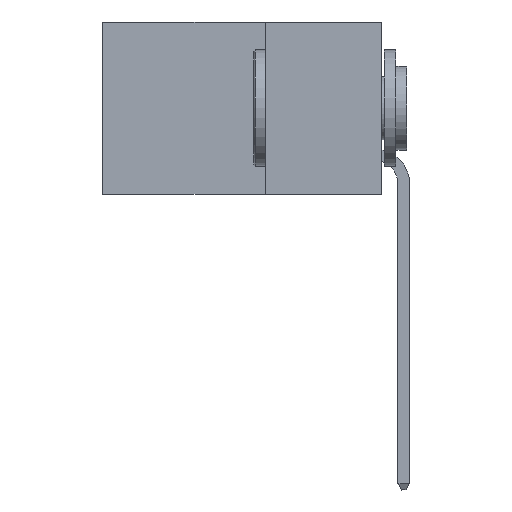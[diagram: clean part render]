
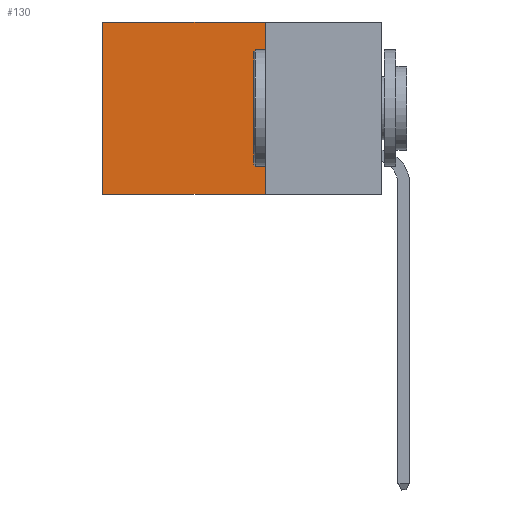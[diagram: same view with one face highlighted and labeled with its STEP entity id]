
A CAD part, left-side view. The second image highlights one B-rep face of the part: STEP entity #130.
In plain terms, the highlighted planar face has unit normal (-1, 0, 0).
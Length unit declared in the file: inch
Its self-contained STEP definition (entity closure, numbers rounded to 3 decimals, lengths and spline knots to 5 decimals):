
#66 = FACE_OUTER_BOUND ( 'NONE', #1054, .T. ) ;
#108 = CARTESIAN_POINT ( 'NONE',  ( 0.2875, 0.6, -0.37 ) ) ;
#113 = DIRECTION ( 'NONE',  ( 0., 1., 0. ) ) ;
#130 = ADVANCED_FACE ( 'NONE', ( #66 ), #8035, .F. ) ;
#578 = LINE ( 'NONE', #3167, #718 ) ;
#718 = VECTOR ( 'NONE', #9207, 39.37008 ) ;
#1054 = EDGE_LOOP ( 'NONE', ( #7247, #6273, #2161, #7801 ) ) ;
#1156 = CARTESIAN_POINT ( 'NONE',  ( 0.2875, 0.25, 0. ) ) ;
#1297 = EDGE_CURVE ( 'NONE', #5763, #5874, #578, .T. ) ;
#1382 = CARTESIAN_POINT ( 'NONE',  ( 0.2875, 0.25, -0.37 ) ) ;
#2161 = ORIENTED_EDGE ( 'NONE', *, *, #1297, .F. ) ;
#2549 = CARTESIAN_POINT ( 'NONE',  ( 0.2875, 0.25, -0.37 ) ) ;
#3167 = CARTESIAN_POINT ( 'NONE',  ( 0.2875, 0.25, 0. ) ) ;
#3944 = CARTESIAN_POINT ( 'NONE',  ( 0.2875, 0.25, 0. ) ) ;
#4031 = LINE ( 'NONE', #5325, #8685 ) ;
#4198 = VERTEX_POINT ( 'NONE', #108 ) ;
#4256 = DIRECTION ( 'NONE',  ( 0., 1., 0. ) ) ;
#4921 = VECTOR ( 'NONE', #7997, 39.37008 ) ;
#5325 = CARTESIAN_POINT ( 'NONE',  ( 0.2875, 0.25, 0. ) ) ;
#5652 = LINE ( 'NONE', #2549, #8105 ) ;
#5763 = VERTEX_POINT ( 'NONE', #3944 ) ;
#5874 = VERTEX_POINT ( 'NONE', #1382 ) ;
#6143 = CARTESIAN_POINT ( 'NONE',  ( 0.2875, 0.6, 0. ) ) ;
#6191 = EDGE_CURVE ( 'NONE', #7496, #4198, #11227, .T. ) ;
#6273 = ORIENTED_EDGE ( 'NONE', *, *, #10768, .F. ) ;
#7247 = ORIENTED_EDGE ( 'NONE', *, *, #6191, .T. ) ;
#7496 = VERTEX_POINT ( 'NONE', #8692 ) ;
#7665 = DIRECTION ( 'NONE',  ( 1., 0., 0. ) ) ;
#7801 = ORIENTED_EDGE ( 'NONE', *, *, #9437, .T. ) ;
#7997 = DIRECTION ( 'NONE',  ( 0., 0., -1. ) ) ;
#8035 = PLANE ( 'NONE',  #9555 ) ;
#8105 = VECTOR ( 'NONE', #4256, 39.37008 ) ;
#8685 = VECTOR ( 'NONE', #113, 39.37008 ) ;
#8692 = CARTESIAN_POINT ( 'NONE',  ( 0.2875, 0.6, 0. ) ) ;
#9207 = DIRECTION ( 'NONE',  ( 0., 0., -1. ) ) ;
#9437 = EDGE_CURVE ( 'NONE', #5763, #7496, #4031, .T. ) ;
#9555 = AXIS2_PLACEMENT_3D ( 'NONE', #1156, #7665, #11287 ) ;
#10768 = EDGE_CURVE ( 'NONE', #5874, #4198, #5652, .T. ) ;
#11227 = LINE ( 'NONE', #6143, #4921 ) ;
#11287 = DIRECTION ( 'NONE',  ( 0., 0., -1. ) ) ;
